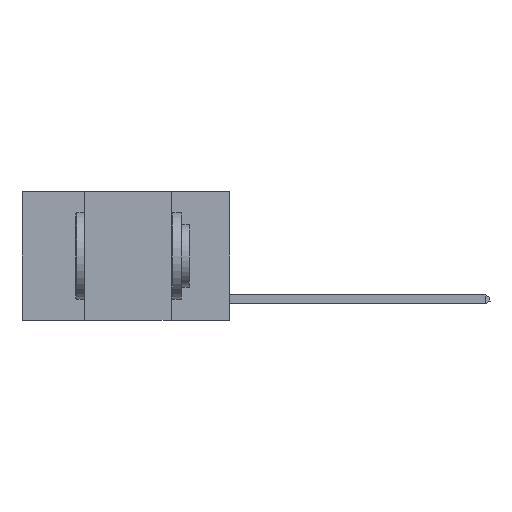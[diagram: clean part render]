
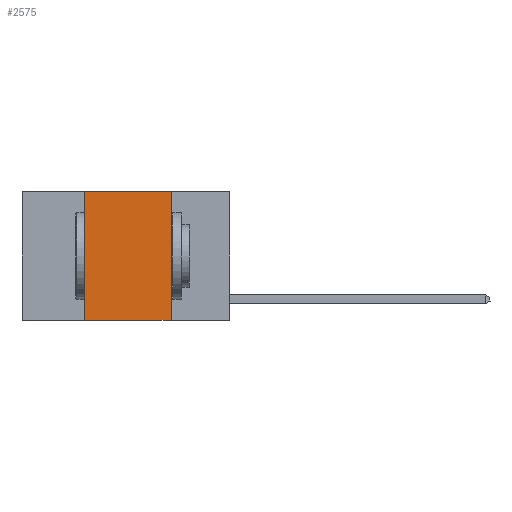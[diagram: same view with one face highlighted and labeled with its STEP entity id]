
A CAD part, left-side view. The second image highlights one B-rep face of the part: STEP entity #2575.
In plain terms, the highlighted planar face has unit normal (-1, 0, 0).
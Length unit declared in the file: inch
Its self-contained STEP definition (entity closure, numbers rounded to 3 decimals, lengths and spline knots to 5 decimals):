
#66 = ORIENTED_EDGE ( 'NONE', *, *, #14495, .F. ) ;
#227 = CARTESIAN_POINT ( 'NONE',  ( 0., 0.17, 0. ) ) ;
#299 = CARTESIAN_POINT ( 'NONE',  ( 0., 0.6, 0. ) ) ;
#1133 = DIRECTION ( 'NONE',  ( 0., -1., 0. ) ) ;
#1674 = DIRECTION ( 'NONE',  ( 0., -1., 0. ) ) ;
#1962 = VERTEX_POINT ( 'NONE', #12409 ) ;
#2575 = ADVANCED_FACE ( 'NONE', ( #20792 ), #4637, .F. ) ;
#3110 = EDGE_CURVE ( 'NONE', #22824, #25554, #23034, .T. ) ;
#3572 = CARTESIAN_POINT ( 'NONE',  ( 0., 0.42, -0.37 ) ) ;
#3909 = EDGE_LOOP ( 'NONE', ( #66, #22509, #26779, #7972 ) ) ;
#4259 = VECTOR ( 'NONE', #25059, 39.37008 ) ;
#4637 = PLANE ( 'NONE',  #11406 ) ;
#7972 = ORIENTED_EDGE ( 'NONE', *, *, #3110, .T. ) ;
#8879 = LINE ( 'NONE', #9417, #12719 ) ;
#9134 = CARTESIAN_POINT ( 'NONE',  ( 0., 0.6, -0.37 ) ) ;
#9417 = CARTESIAN_POINT ( 'NONE',  ( 0., 0.6, 0. ) ) ;
#10697 = VERTEX_POINT ( 'NONE', #19329 ) ;
#11406 = AXIS2_PLACEMENT_3D ( 'NONE', #299, #20930, #16692 ) ;
#11990 = CARTESIAN_POINT ( 'NONE',  ( 0., 0.42, 0. ) ) ;
#12409 = CARTESIAN_POINT ( 'NONE',  ( 0., 0.42, 0. ) ) ;
#12719 = VECTOR ( 'NONE', #1674, 39.37008 ) ;
#14173 = CARTESIAN_POINT ( 'NONE',  ( 0., 0.17, -0.37 ) ) ;
#14495 = EDGE_CURVE ( 'NONE', #10697, #25554, #16623, .T. ) ;
#16165 = DIRECTION ( 'NONE',  ( 0., 0., 1. ) ) ;
#16623 = LINE ( 'NONE', #227, #4259 ) ;
#16692 = DIRECTION ( 'NONE',  ( 0., 0., -1. ) ) ;
#18456 = EDGE_CURVE ( 'NONE', #22824, #1962, #24322, .T. ) ;
#18712 = VECTOR ( 'NONE', #1133, 39.37008 ) ;
#19329 = CARTESIAN_POINT ( 'NONE',  ( 0., 0.17, 0. ) ) ;
#19546 = VECTOR ( 'NONE', #16165, 39.37008 ) ;
#20792 = FACE_OUTER_BOUND ( 'NONE', #3909, .T. ) ;
#20930 = DIRECTION ( 'NONE',  ( 1., 0., 0. ) ) ;
#22509 = ORIENTED_EDGE ( 'NONE', *, *, #23967, .F. ) ;
#22824 = VERTEX_POINT ( 'NONE', #3572 ) ;
#23034 = LINE ( 'NONE', #9134, #18712 ) ;
#23967 = EDGE_CURVE ( 'NONE', #1962, #10697, #8879, .T. ) ;
#24322 = LINE ( 'NONE', #11990, #19546 ) ;
#25059 = DIRECTION ( 'NONE',  ( 0., 0., -1. ) ) ;
#25554 = VERTEX_POINT ( 'NONE', #14173 ) ;
#26779 = ORIENTED_EDGE ( 'NONE', *, *, #18456, .F. ) ;
